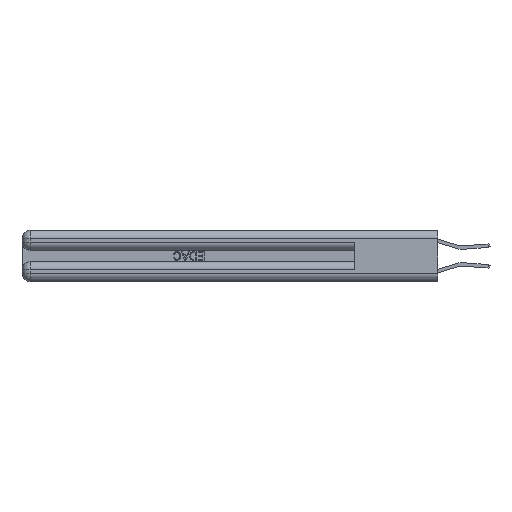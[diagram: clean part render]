
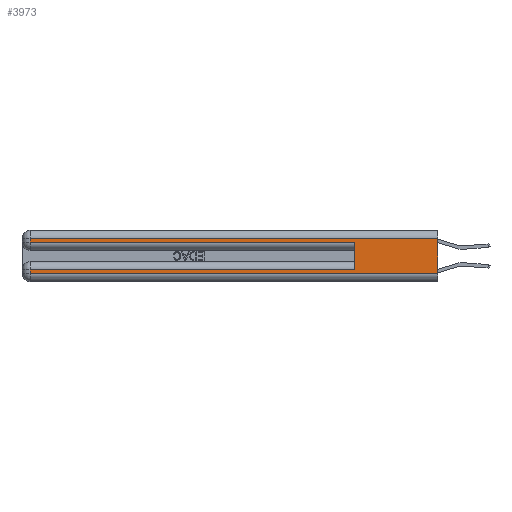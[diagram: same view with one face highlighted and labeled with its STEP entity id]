
A CAD part, left-side view. The second image highlights one B-rep face of the part: STEP entity #3973.
In plain terms, the highlighted planar face has unit normal (-1, 0, 0).
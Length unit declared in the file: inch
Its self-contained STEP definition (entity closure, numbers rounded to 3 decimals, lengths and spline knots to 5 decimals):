
#657 = VERTEX_POINT ( 'NONE', #25446 ) ;
#662 = CARTESIAN_POINT ( 'NONE',  ( 0., 2.94, 0.37 ) ) ;
#1780 = ORIENTED_EDGE ( 'NONE', *, *, #21178, .F. ) ;
#2933 = ORIENTED_EDGE ( 'NONE', *, *, #6745, .T. ) ;
#2950 = CARTESIAN_POINT ( 'NONE',  ( 0., 2.94, 0.31 ) ) ;
#3105 = EDGE_CURVE ( 'NONE', #8435, #6396, #27303, .T. ) ;
#3172 = DIRECTION ( 'NONE',  ( 0., -1., 0. ) ) ;
#3207 = FACE_OUTER_BOUND ( 'NONE', #16132, .T. ) ;
#3262 = CARTESIAN_POINT ( 'NONE',  ( 0., 2.94, 0.06 ) ) ;
#3705 = CARTESIAN_POINT ( 'NONE',  ( 0., 0., 0.06 ) ) ;
#3973 = ADVANCED_FACE ( 'NONE', ( #3207 ), #10067, .F. ) ;
#4595 = CARTESIAN_POINT ( 'NONE',  ( 0., 0., 0.085 ) ) ;
#4681 = ORIENTED_EDGE ( 'NONE', *, *, #14891, .T. ) ;
#5341 = VECTOR ( 'NONE', #15320, 39.37008 ) ;
#6396 = VERTEX_POINT ( 'NONE', #14847 ) ;
#6449 = CARTESIAN_POINT ( 'NONE',  ( 0., 2.94, 0.285 ) ) ;
#6745 = EDGE_CURVE ( 'NONE', #6396, #7273, #9601, .T. ) ;
#7273 = VERTEX_POINT ( 'NONE', #3262 ) ;
#8435 = VERTEX_POINT ( 'NONE', #9291 ) ;
#8777 = CARTESIAN_POINT ( 'NONE',  ( 0., 0., 0.31 ) ) ;
#9013 = VECTOR ( 'NONE', #17683, 39.37008 ) ;
#9143 = DIRECTION ( 'NONE',  ( 0., 1., 0. ) ) ;
#9291 = CARTESIAN_POINT ( 'NONE',  ( 0., 0.6, 0.085 ) ) ;
#9440 = ORIENTED_EDGE ( 'NONE', *, *, #11431, .T. ) ;
#9601 = LINE ( 'NONE', #662, #26351 ) ;
#9692 = VERTEX_POINT ( 'NONE', #6449 ) ;
#10067 = PLANE ( 'NONE',  #10561 ) ;
#10561 = AXIS2_PLACEMENT_3D ( 'NONE', #19160, #17954, #17507 ) ;
#10760 = VERTEX_POINT ( 'NONE', #2950 ) ;
#11431 = EDGE_CURVE ( 'NONE', #19590, #10760, #20494, .T. ) ;
#11486 = CARTESIAN_POINT ( 'NONE',  ( 0., 0., 0.37 ) ) ;
#11746 = EDGE_CURVE ( 'NONE', #9692, #22724, #14507, .T. ) ;
#11792 = VECTOR ( 'NONE', #20575, 39.37008 ) ;
#11894 = CARTESIAN_POINT ( 'NONE',  ( 0., 2.94, 0.37 ) ) ;
#12008 = ORIENTED_EDGE ( 'NONE', *, *, #11746, .T. ) ;
#12039 = DIRECTION ( 'NONE',  ( 0., 0., -1. ) ) ;
#12186 = LINE ( 'NONE', #11894, #28105 ) ;
#12952 = ORIENTED_EDGE ( 'NONE', *, *, #13865, .F. ) ;
#13865 = EDGE_CURVE ( 'NONE', #19590, #657, #27622, .T. ) ;
#13964 = CARTESIAN_POINT ( 'NONE',  ( 0., 0.6, 0.285 ) ) ;
#14507 = LINE ( 'NONE', #23626, #27509 ) ;
#14847 = CARTESIAN_POINT ( 'NONE',  ( 0., 2.94, 0.085 ) ) ;
#14891 = EDGE_CURVE ( 'NONE', #10760, #9692, #12186, .T. ) ;
#15320 = DIRECTION ( 'NONE',  ( 0., -1., 0. ) ) ;
#16021 = DIRECTION ( 'NONE',  ( 0., 0., -1. ) ) ;
#16132 = EDGE_LOOP ( 'NONE', ( #12952, #9440, #4681, #12008, #1780, #25778, #2933, #16923 ) ) ;
#16923 = ORIENTED_EDGE ( 'NONE', *, *, #24012, .T. ) ;
#17507 = DIRECTION ( 'NONE',  ( 0., 0., -1. ) ) ;
#17683 = DIRECTION ( 'NONE',  ( 0., 0., 1. ) ) ;
#17954 = DIRECTION ( 'NONE',  ( 1., 0., 0. ) ) ;
#18898 = VECTOR ( 'NONE', #9143, 39.37008 ) ;
#19160 = CARTESIAN_POINT ( 'NONE',  ( 0., 0., 0.37 ) ) ;
#19590 = VERTEX_POINT ( 'NONE', #8777 ) ;
#19927 = LINE ( 'NONE', #22319, #9013 ) ;
#20494 = LINE ( 'NONE', #24839, #18898 ) ;
#20575 = DIRECTION ( 'NONE',  ( 0., 0., -1. ) ) ;
#21178 = EDGE_CURVE ( 'NONE', #8435, #22724, #19927, .T. ) ;
#21758 = LINE ( 'NONE', #3705, #5341 ) ;
#22319 = CARTESIAN_POINT ( 'NONE',  ( 0., 0.6, 0.145 ) ) ;
#22429 = VECTOR ( 'NONE', #26850, 39.37008 ) ;
#22724 = VERTEX_POINT ( 'NONE', #13964 ) ;
#23626 = CARTESIAN_POINT ( 'NONE',  ( 0., 0., 0.285 ) ) ;
#24012 = EDGE_CURVE ( 'NONE', #7273, #657, #21758, .T. ) ;
#24839 = CARTESIAN_POINT ( 'NONE',  ( 0., 0., 0.31 ) ) ;
#25446 = CARTESIAN_POINT ( 'NONE',  ( 0., 0., 0.06 ) ) ;
#25778 = ORIENTED_EDGE ( 'NONE', *, *, #3105, .T. ) ;
#26351 = VECTOR ( 'NONE', #16021, 39.37008 ) ;
#26850 = DIRECTION ( 'NONE',  ( 0., 1., 0. ) ) ;
#27303 = LINE ( 'NONE', #4595, #22429 ) ;
#27509 = VECTOR ( 'NONE', #3172, 39.37008 ) ;
#27622 = LINE ( 'NONE', #11486, #11792 ) ;
#28105 = VECTOR ( 'NONE', #12039, 39.37008 ) ;
